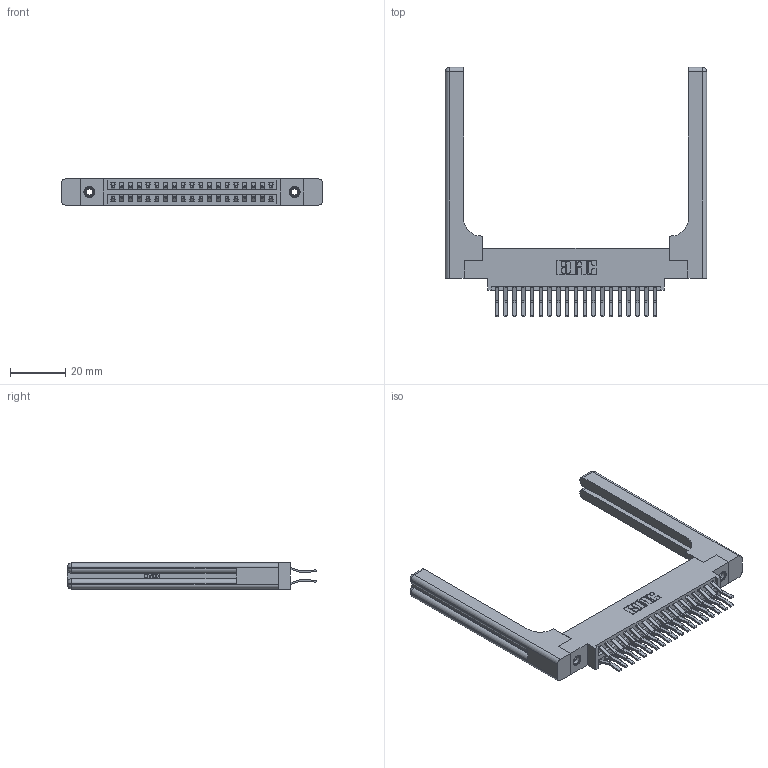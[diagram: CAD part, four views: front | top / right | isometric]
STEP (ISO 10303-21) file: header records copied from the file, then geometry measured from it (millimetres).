
FILE_DESCRIPTION (( 'STEP AP203' ), '1' );
FILE_NAME ('396-038-560-858.STEP', '2019-11-02T05:38:28', ( '' ), ( '' ), 'SwSTEP 2.0', 'SolidWorks 2016', '' );
FILE_SCHEMA (( 'CONFIG_CONTROL_DESIGN' ));
Length unit declared in the file: inch
Products named in the file (5): 346 Part_0.170 Offset - 0.156 Dia-TH; 345-292-001_560 Tail; 345-250-001_345-250-001-102; 346-220-058_345-220-058; 396-038-560-858
Assembly tree (43 placements, depth 2):
  396-038-560-858
    346 Part_0.170 Offset - 0.156 Dia-TH
    345-292-001_560 Tail  x38
    345-250-001_345-250-001-102  x2
    346-220-058_345-220-058  x2
Bounding box: 94.39 x 90.05 x 9.4 mm (x, y, z)
Volume: 16613.9 mm3; surface area: 17991 mm2
Topology: 43 solids, 43 shells, 2434 faces, 7125 edges, 4678 vertices
Faces by surface type: plane 1558, cylinder 816, bspline 36, cone 12, sphere 8, torus 4
Entity records: 20898 total; most frequent: CARTESIAN_POINT 4485, ORIENTED_EDGE 3216, DIRECTION 2940, EDGE_CURVE 1608, LINE 1304, VECTOR 1304, VERTEX_POINT 1062, AXIS2_PLACEMENT_3D 818
